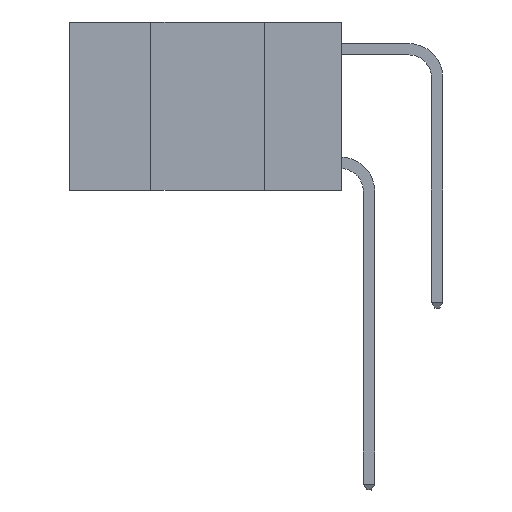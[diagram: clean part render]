
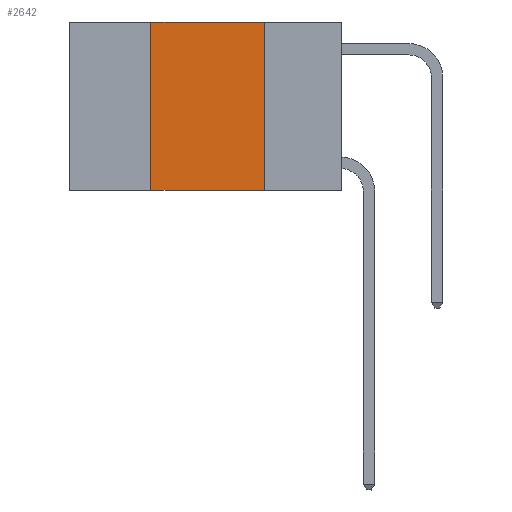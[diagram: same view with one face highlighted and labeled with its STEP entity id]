
A CAD part, left-side view. The second image highlights one B-rep face of the part: STEP entity #2642.
In plain terms, the highlighted planar face has unit normal (-1, 0, 0).
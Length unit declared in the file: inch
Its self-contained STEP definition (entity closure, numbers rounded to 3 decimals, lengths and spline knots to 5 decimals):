
#441 = ORIENTED_EDGE ( 'NONE', *, *, #3544, .F. ) ;
#788 = ORIENTED_EDGE ( 'NONE', *, *, #10293, .T. ) ;
#1912 = LINE ( 'NONE', #20167, #7744 ) ;
#1953 = EDGE_CURVE ( 'NONE', #2878, #16985, #6257, .T. ) ;
#2642 = ADVANCED_FACE ( 'NONE', ( #23316 ), #7709, .F. ) ;
#2878 = VERTEX_POINT ( 'NONE', #21252 ) ;
#3544 = EDGE_CURVE ( 'NONE', #16985, #26304, #19813, .T. ) ;
#3689 = VECTOR ( 'NONE', #9796, 39.37008 ) ;
#6257 = LINE ( 'NONE', #21836, #15954 ) ;
#7709 = PLANE ( 'NONE',  #31388 ) ;
#7744 = VECTOR ( 'NONE', #12191, 39.37008 ) ;
#8291 = VERTEX_POINT ( 'NONE', #26374 ) ;
#8765 = ORIENTED_EDGE ( 'NONE', *, *, #12159, .F. ) ;
#8821 = CARTESIAN_POINT ( 'NONE',  ( 0., 0.17, -0.37 ) ) ;
#9796 = DIRECTION ( 'NONE',  ( 0., 0., -1. ) ) ;
#10293 = EDGE_CURVE ( 'NONE', #8291, #26304, #29683, .T. ) ;
#10416 = DIRECTION ( 'NONE',  ( 1., 0., 0. ) ) ;
#11461 = VECTOR ( 'NONE', #29341, 39.37008 ) ;
#12159 = EDGE_CURVE ( 'NONE', #8291, #2878, #1912, .T. ) ;
#12191 = DIRECTION ( 'NONE',  ( 0., 0., 1. ) ) ;
#15954 = VECTOR ( 'NONE', #26889, 39.37008 ) ;
#16985 = VERTEX_POINT ( 'NONE', #25119 ) ;
#17761 = CARTESIAN_POINT ( 'NONE',  ( 0., 0.17, 0. ) ) ;
#18053 = CARTESIAN_POINT ( 'NONE',  ( 0., 0.6, 0. ) ) ;
#19813 = LINE ( 'NONE', #17761, #3689 ) ;
#20167 = CARTESIAN_POINT ( 'NONE',  ( 0., 0.42, 0. ) ) ;
#21252 = CARTESIAN_POINT ( 'NONE',  ( 0., 0.42, 0. ) ) ;
#21836 = CARTESIAN_POINT ( 'NONE',  ( 0., 0.6, 0. ) ) ;
#23316 = FACE_OUTER_BOUND ( 'NONE', #26663, .T. ) ;
#25119 = CARTESIAN_POINT ( 'NONE',  ( 0., 0.17, 0. ) ) ;
#26304 = VERTEX_POINT ( 'NONE', #8821 ) ;
#26374 = CARTESIAN_POINT ( 'NONE',  ( 0., 0.42, -0.37 ) ) ;
#26663 = EDGE_LOOP ( 'NONE', ( #441, #29354, #8765, #788 ) ) ;
#26889 = DIRECTION ( 'NONE',  ( 0., -1., 0. ) ) ;
#29341 = DIRECTION ( 'NONE',  ( 0., -1., 0. ) ) ;
#29354 = ORIENTED_EDGE ( 'NONE', *, *, #1953, .F. ) ;
#29683 = LINE ( 'NONE', #32393, #11461 ) ;
#31230 = DIRECTION ( 'NONE',  ( 0., 0., -1. ) ) ;
#31388 = AXIS2_PLACEMENT_3D ( 'NONE', #18053, #10416, #31230 ) ;
#32393 = CARTESIAN_POINT ( 'NONE',  ( 0., 0.6, -0.37 ) ) ;
